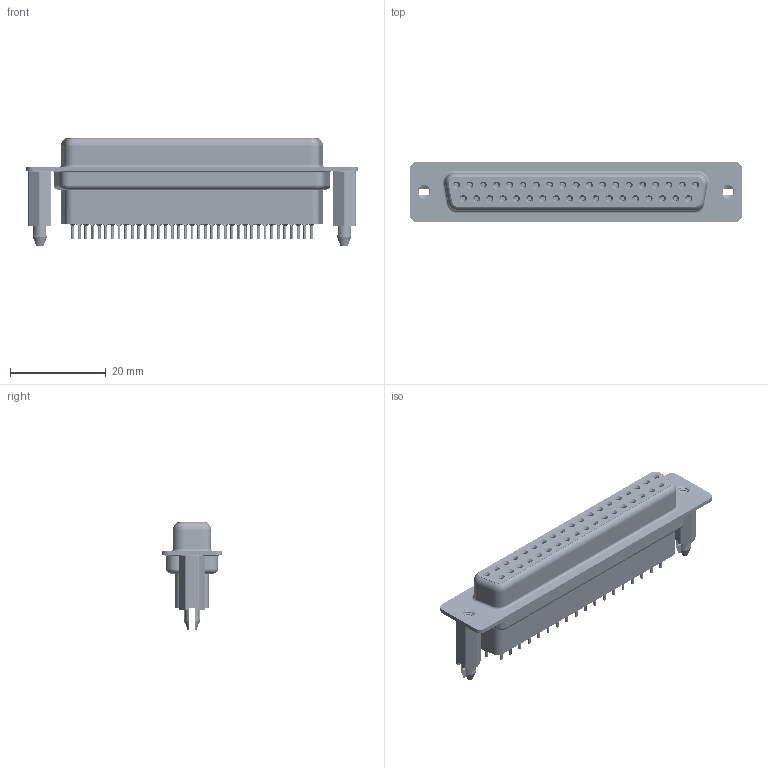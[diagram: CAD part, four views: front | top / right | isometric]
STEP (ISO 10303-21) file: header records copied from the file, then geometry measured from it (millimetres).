
FILE_DESCRIPTION (( 'STEP AP203' ), '1' );
FILE_NAME ('628-037-621-556.STEP', '2018-10-20T05:04:45', ( '' ), ( '' ), 'SwSTEP 2.0', 'SolidWorks 2016', '' );
FILE_SCHEMA (( 'CONFIG_CONTROL_DESIGN' ));
Length unit declared in the file: millimetre
Products named in the file (7): 628 Housing_37 HP; 628 Shell Front_37 Contacts; 628 Shell Rear_37 Contacts; 628 Contact Row 1_21H; 628 Contact Row 2_21H; 628 4-40 Threaded Boardlock_HP; 628-037-621-556
Assembly tree (42 placements, depth 2):
  628-037-621-556
    628 Housing_37 HP
    628 Shell Front_37 Contacts
    628 Shell Rear_37 Contacts
    628 Contact Row 1_21H  x19
    628 Contact Row 2_21H  x18
    628 4-40 Threaded Boardlock_HP  x2
Bounding box: 69.3 x 12.6 x 22.4 mm (x, y, z)
Volume: 7819.1 mm3; surface area: 17416.7 mm2
Topology: 42 solids, 42 shells, 4911 faces, 12648 edges, 7905 vertices
Faces by surface type: cylinder 1411, plane 1243, torus 940, bspline 746, cone 571
Entity records: 34443 total; most frequent: CARTESIAN_POINT 9744, DIRECTION 5080, ORIENTED_EDGE 4632, EDGE_CURVE 2316, AXIS2_PLACEMENT_3D 2123, VERTEX_POINT 1474, EDGE_LOOP 1180, CIRCLE 1147
